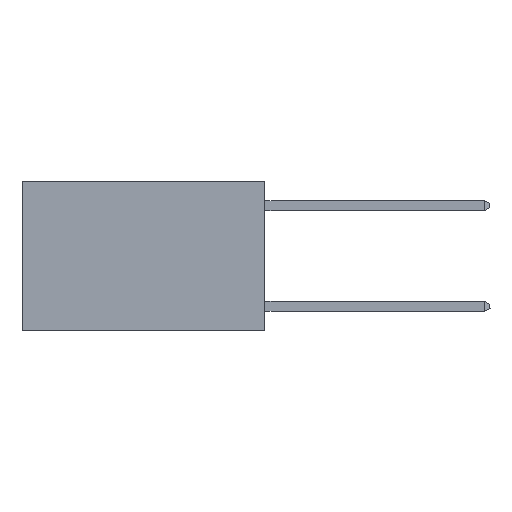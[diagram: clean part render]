
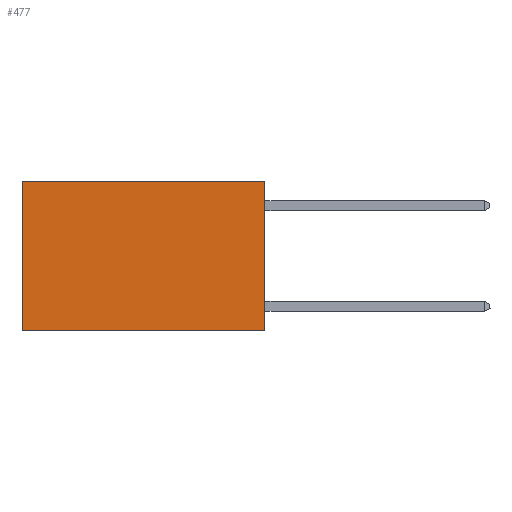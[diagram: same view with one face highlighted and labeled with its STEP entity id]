
A CAD part, left-side view. The second image highlights one B-rep face of the part: STEP entity #477.
In plain terms, the highlighted planar face has unit normal (-1, 0, 0).
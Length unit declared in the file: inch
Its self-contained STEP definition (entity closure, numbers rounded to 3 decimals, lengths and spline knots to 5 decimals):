
#477 = ADVANCED_FACE ( 'NONE', ( #13571 ), #6109, .F. ) ;
#1035 = VECTOR ( 'NONE', #1055, 39.37008 ) ;
#1055 = DIRECTION ( 'NONE',  ( 0., 0., -1. ) ) ;
#2850 = VERTEX_POINT ( 'NONE', #5833 ) ;
#3656 = CARTESIAN_POINT ( 'NONE',  ( 0.2625, 0.6, 0. ) ) ;
#3798 = AXIS2_PLACEMENT_3D ( 'NONE', #12886, #3912, #11264 ) ;
#3912 = DIRECTION ( 'NONE',  ( 1., 0., 0. ) ) ;
#5055 = LINE ( 'NONE', #5807, #14914 ) ;
#5807 = CARTESIAN_POINT ( 'NONE',  ( 0.2625, 0., 0. ) ) ;
#5833 = CARTESIAN_POINT ( 'NONE',  ( 0.2625, 0., -0.37 ) ) ;
#6006 = DIRECTION ( 'NONE',  ( 0., 1., 0. ) ) ;
#6070 = ORIENTED_EDGE ( 'NONE', *, *, #7068, .F. ) ;
#6109 = PLANE ( 'NONE',  #3798 ) ;
#6641 = ORIENTED_EDGE ( 'NONE', *, *, #12433, .T. ) ;
#7068 = EDGE_CURVE ( 'NONE', #14791, #2850, #5055, .T. ) ;
#7604 = LINE ( 'NONE', #10210, #1035 ) ;
#7856 = EDGE_CURVE ( 'NONE', #2850, #10683, #9104, .T. ) ;
#8441 = DIRECTION ( 'NONE',  ( 0., 0., -1. ) ) ;
#8488 = VECTOR ( 'NONE', #16246, 39.37008 ) ;
#9104 = LINE ( 'NONE', #9888, #10086 ) ;
#9475 = EDGE_CURVE ( 'NONE', #14509, #10683, #7604, .T. ) ;
#9888 = CARTESIAN_POINT ( 'NONE',  ( 0.2625, 0., -0.37 ) ) ;
#10086 = VECTOR ( 'NONE', #6006, 39.37008 ) ;
#10210 = CARTESIAN_POINT ( 'NONE',  ( 0.2625, 0.6, 0. ) ) ;
#10683 = VERTEX_POINT ( 'NONE', #15086 ) ;
#11264 = DIRECTION ( 'NONE',  ( 0., 0., -1. ) ) ;
#11909 = CARTESIAN_POINT ( 'NONE',  ( 0.2625, 0., 0. ) ) ;
#12433 = EDGE_CURVE ( 'NONE', #14791, #14509, #14887, .T. ) ;
#12886 = CARTESIAN_POINT ( 'NONE',  ( 0.2625, 0., 0. ) ) ;
#13571 = FACE_OUTER_BOUND ( 'NONE', #15304, .T. ) ;
#14039 = ORIENTED_EDGE ( 'NONE', *, *, #9475, .T. ) ;
#14506 = ORIENTED_EDGE ( 'NONE', *, *, #7856, .F. ) ;
#14509 = VERTEX_POINT ( 'NONE', #3656 ) ;
#14791 = VERTEX_POINT ( 'NONE', #11909 ) ;
#14887 = LINE ( 'NONE', #14938, #8488 ) ;
#14914 = VECTOR ( 'NONE', #8441, 39.37008 ) ;
#14938 = CARTESIAN_POINT ( 'NONE',  ( 0.2625, 0., 0. ) ) ;
#15086 = CARTESIAN_POINT ( 'NONE',  ( 0.2625, 0.6, -0.37 ) ) ;
#15304 = EDGE_LOOP ( 'NONE', ( #14039, #14506, #6070, #6641 ) ) ;
#16246 = DIRECTION ( 'NONE',  ( 0., 1., 0. ) ) ;
